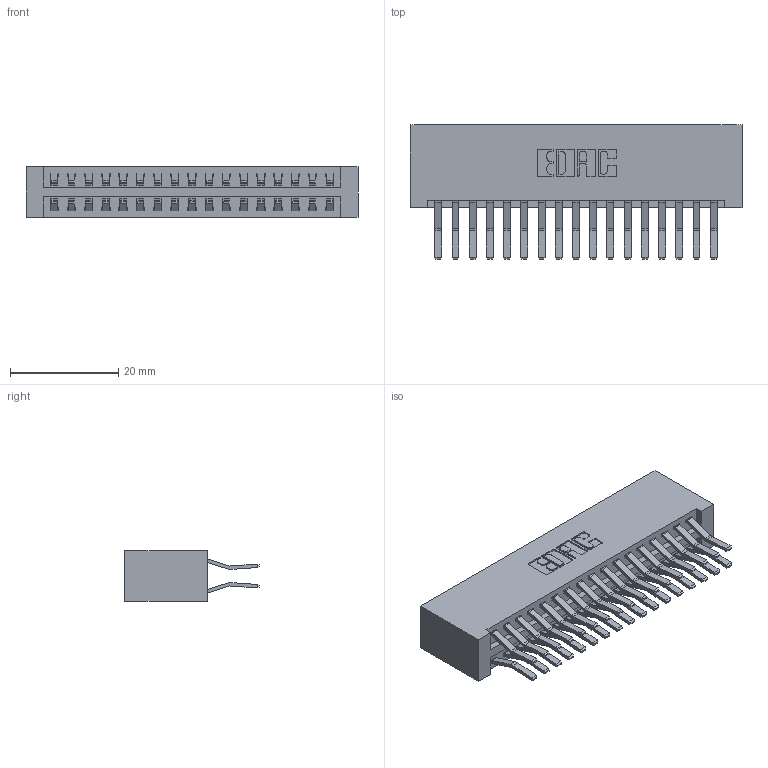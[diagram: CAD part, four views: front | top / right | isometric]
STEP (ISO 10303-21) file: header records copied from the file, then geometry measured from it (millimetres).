
FILE_DESCRIPTION (( 'STEP AP203' ), '1' );
FILE_NAME ('346-034-560-201.STEP', '2022-05-19T20:36:13', ( '' ), ( '' ), 'SwSTEP 2.0', 'SolidWorks 2020', '' );
FILE_SCHEMA (( 'CONFIG_CONTROL_DESIGN' ));
Length unit declared in the file: inch
Products named in the file (3): 346-034-560-201; 346 Part_No Mounting Lugs; 345-292-001_560 Tail
Assembly tree (35 placements, depth 2):
  346-034-560-201
    346 Part_No Mounting Lugs
    345-292-001_560 Tail  x34
Bounding box: 61.21 x 24.78 x 9.4 mm (x, y, z)
Volume: 6571.1 mm3; surface area: 9397.2 mm2
Topology: 35 solids, 35 shells, 1950 faces, 5779 edges, 3806 vertices
Faces by surface type: plane 1262, cylinder 688
Entity records: 14271 total; most frequent: CARTESIAN_POINT 2384, ORIENTED_EDGE 2318, DIRECTION 2151, EDGE_CURVE 1159, VECTOR 963, LINE 963, VERTEX_POINT 770, AXIS2_PLACEMENT_3D 594
